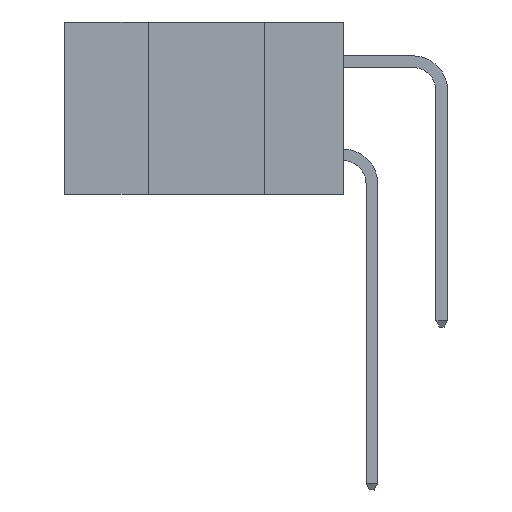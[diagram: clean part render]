
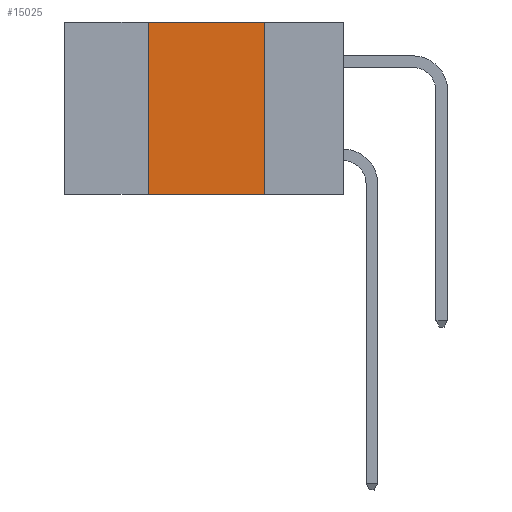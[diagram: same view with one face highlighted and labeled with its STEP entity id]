
A CAD part, left-side view. The second image highlights one B-rep face of the part: STEP entity #15025.
In plain terms, the highlighted planar face has unit normal (-1, 0, 0).
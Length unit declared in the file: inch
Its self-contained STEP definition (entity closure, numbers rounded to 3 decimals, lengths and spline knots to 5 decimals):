
#42 = ORIENTED_EDGE ( 'NONE', *, *, #19988, .F. ) ;
#171 = VERTEX_POINT ( 'NONE', #1491 ) ;
#1012 = CARTESIAN_POINT ( 'NONE',  ( 0., 0.17, 0. ) ) ;
#1491 = CARTESIAN_POINT ( 'NONE',  ( 0., 0.42, 0. ) ) ;
#2945 = CARTESIAN_POINT ( 'NONE',  ( 0., 0.42, 0. ) ) ;
#3090 = EDGE_CURVE ( 'NONE', #18724, #14207, #17441, .T. ) ;
#3771 = VERTEX_POINT ( 'NONE', #4696 ) ;
#4166 = CARTESIAN_POINT ( 'NONE',  ( 0., 0.6, 0. ) ) ;
#4295 = LINE ( 'NONE', #2945, #12111 ) ;
#4696 = CARTESIAN_POINT ( 'NONE',  ( 0., 0.42, -0.37 ) ) ;
#5805 = DIRECTION ( 'NONE',  ( 0., -1., 0. ) ) ;
#8398 = CARTESIAN_POINT ( 'NONE',  ( 0., 0.17, -0.37 ) ) ;
#8666 = ORIENTED_EDGE ( 'NONE', *, *, #3090, .F. ) ;
#8747 = DIRECTION ( 'NONE',  ( 1., 0., 0. ) ) ;
#8943 = FACE_OUTER_BOUND ( 'NONE', #14192, .T. ) ;
#9682 = ORIENTED_EDGE ( 'NONE', *, *, #15040, .T. ) ;
#10875 = CARTESIAN_POINT ( 'NONE',  ( 0., 0.17, 0. ) ) ;
#11044 = ORIENTED_EDGE ( 'NONE', *, *, #13744, .F. ) ;
#11836 = CARTESIAN_POINT ( 'NONE',  ( 0., 0.6, -0.37 ) ) ;
#11905 = DIRECTION ( 'NONE',  ( 0., -1., 0. ) ) ;
#12111 = VECTOR ( 'NONE', #20045, 39.37008 ) ;
#12587 = LINE ( 'NONE', #11836, #17756 ) ;
#12651 = AXIS2_PLACEMENT_3D ( 'NONE', #19847, #8747, #16633 ) ;
#13744 = EDGE_CURVE ( 'NONE', #171, #18724, #16614, .T. ) ;
#14192 = EDGE_LOOP ( 'NONE', ( #8666, #11044, #42, #9682 ) ) ;
#14207 = VERTEX_POINT ( 'NONE', #8398 ) ;
#15025 = ADVANCED_FACE ( 'NONE', ( #8943 ), #19708, .F. ) ;
#15040 = EDGE_CURVE ( 'NONE', #3771, #14207, #12587, .T. ) ;
#15965 = VECTOR ( 'NONE', #17162, 39.37008 ) ;
#16614 = LINE ( 'NONE', #4166, #17815 ) ;
#16633 = DIRECTION ( 'NONE',  ( 0., 0., -1. ) ) ;
#17162 = DIRECTION ( 'NONE',  ( 0., 0., -1. ) ) ;
#17441 = LINE ( 'NONE', #10875, #15965 ) ;
#17756 = VECTOR ( 'NONE', #11905, 39.37008 ) ;
#17815 = VECTOR ( 'NONE', #5805, 39.37008 ) ;
#18724 = VERTEX_POINT ( 'NONE', #1012 ) ;
#19708 = PLANE ( 'NONE',  #12651 ) ;
#19847 = CARTESIAN_POINT ( 'NONE',  ( 0., 0.6, 0. ) ) ;
#19988 = EDGE_CURVE ( 'NONE', #3771, #171, #4295, .T. ) ;
#20045 = DIRECTION ( 'NONE',  ( 0., 0., 1. ) ) ;
